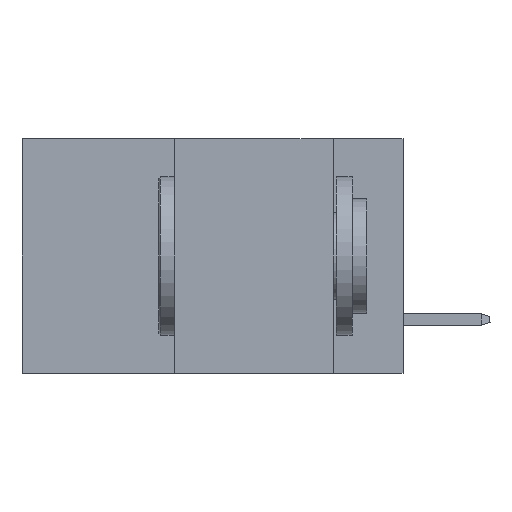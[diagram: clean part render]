
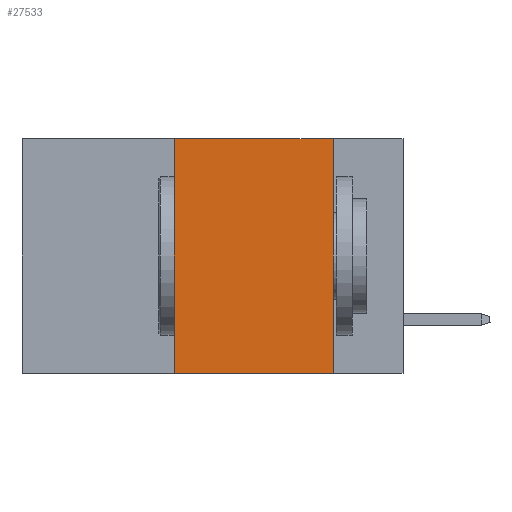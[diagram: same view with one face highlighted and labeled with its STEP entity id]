
A CAD part, left-side view. The second image highlights one B-rep face of the part: STEP entity #27533.
In plain terms, the highlighted planar face has unit normal (-1, 0, 0).
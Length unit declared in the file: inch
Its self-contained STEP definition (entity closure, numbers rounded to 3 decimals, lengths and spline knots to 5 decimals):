
#2528 = ORIENTED_EDGE ( 'NONE', *, *, #12377, .F. ) ;
#3024 = ORIENTED_EDGE ( 'NONE', *, *, #33481, .F. ) ;
#3080 = DIRECTION ( 'NONE',  ( 0., -1., 0. ) ) ;
#4909 = CARTESIAN_POINT ( 'NONE',  ( 0., 0.11, 0. ) ) ;
#7873 = LINE ( 'NONE', #14511, #19024 ) ;
#10731 = VECTOR ( 'NONE', #19237, 39.37008 ) ;
#12377 = EDGE_CURVE ( 'NONE', #17044, #42088, #39205, .T. ) ;
#14511 = CARTESIAN_POINT ( 'NONE',  ( 0., 0.6, 0. ) ) ;
#15942 = ORIENTED_EDGE ( 'NONE', *, *, #31984, .F. ) ;
#16174 = CARTESIAN_POINT ( 'NONE',  ( 0., 0.6, -0.37 ) ) ;
#16259 = CARTESIAN_POINT ( 'NONE',  ( 0., 0.11, -0.37 ) ) ;
#16513 = CARTESIAN_POINT ( 'NONE',  ( 0., 0.11, 0. ) ) ;
#17044 = VERTEX_POINT ( 'NONE', #4909 ) ;
#19024 = VECTOR ( 'NONE', #34420, 39.37008 ) ;
#19237 = DIRECTION ( 'NONE',  ( 0., 0., 1. ) ) ;
#22448 = LINE ( 'NONE', #31468, #10731 ) ;
#23896 = VECTOR ( 'NONE', #3080, 39.37008 ) ;
#25621 = FACE_OUTER_BOUND ( 'NONE', #35864, .T. ) ;
#27533 = ADVANCED_FACE ( 'NONE', ( #25621 ), #32049, .F. ) ;
#29334 = VERTEX_POINT ( 'NONE', #37314 ) ;
#31468 = CARTESIAN_POINT ( 'NONE',  ( 0., 0.36, 0. ) ) ;
#31745 = AXIS2_PLACEMENT_3D ( 'NONE', #41906, #38679, #34832 ) ;
#31984 = EDGE_CURVE ( 'NONE', #29334, #38716, #22448, .T. ) ;
#32049 = PLANE ( 'NONE',  #31745 ) ;
#33481 = EDGE_CURVE ( 'NONE', #38716, #17044, #7873, .T. ) ;
#34420 = DIRECTION ( 'NONE',  ( 0., -1., 0. ) ) ;
#34832 = DIRECTION ( 'NONE',  ( 0., 0., -1. ) ) ;
#35460 = ORIENTED_EDGE ( 'NONE', *, *, #37347, .T. ) ;
#35864 = EDGE_LOOP ( 'NONE', ( #2528, #3024, #15942, #35460 ) ) ;
#36003 = DIRECTION ( 'NONE',  ( 0., 0., -1. ) ) ;
#36077 = CARTESIAN_POINT ( 'NONE',  ( 0., 0.36, 0. ) ) ;
#37314 = CARTESIAN_POINT ( 'NONE',  ( 0., 0.36, -0.37 ) ) ;
#37347 = EDGE_CURVE ( 'NONE', #29334, #42088, #42298, .T. ) ;
#38679 = DIRECTION ( 'NONE',  ( 1., 0., 0. ) ) ;
#38716 = VERTEX_POINT ( 'NONE', #36077 ) ;
#39193 = VECTOR ( 'NONE', #36003, 39.37008 ) ;
#39205 = LINE ( 'NONE', #16513, #39193 ) ;
#41906 = CARTESIAN_POINT ( 'NONE',  ( 0., 0.6, 0. ) ) ;
#42088 = VERTEX_POINT ( 'NONE', #16259 ) ;
#42298 = LINE ( 'NONE', #16174, #23896 ) ;
